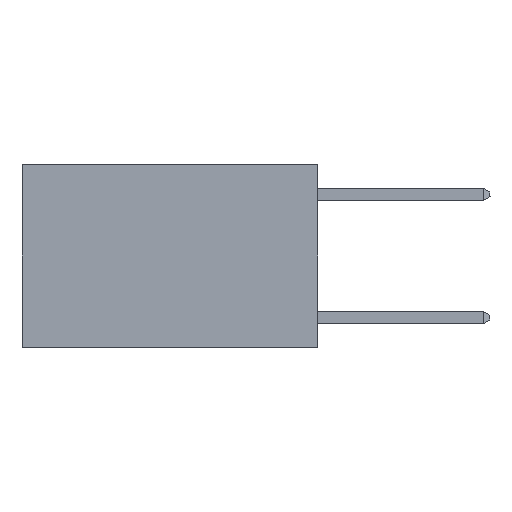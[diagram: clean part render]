
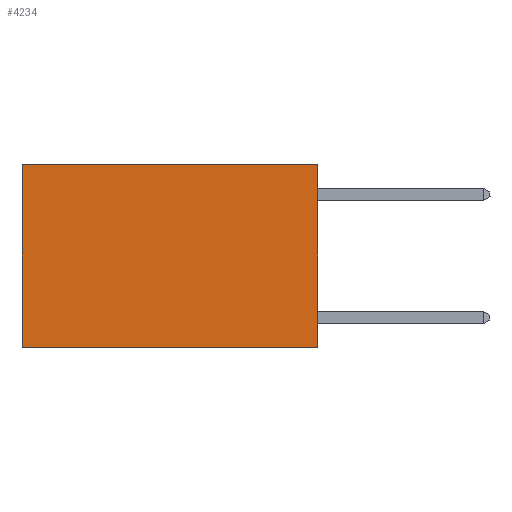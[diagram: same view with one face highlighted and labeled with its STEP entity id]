
A CAD part, left-side view. The second image highlights one B-rep face of the part: STEP entity #4234.
In plain terms, the highlighted planar face has unit normal (-1, 0, 0).
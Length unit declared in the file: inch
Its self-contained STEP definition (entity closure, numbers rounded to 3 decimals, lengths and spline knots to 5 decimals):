
#68 = VECTOR ( 'NONE', #19701, 39.37008 ) ;
#209 = CARTESIAN_POINT ( 'NONE',  ( 0.2625, 0., -0.37 ) ) ;
#572 = EDGE_CURVE ( 'NONE', #8072, #10551, #11175, .T. ) ;
#1167 = LINE ( 'NONE', #19522, #68 ) ;
#1258 = PLANE ( 'NONE',  #15353 ) ;
#1489 = DIRECTION ( 'NONE',  ( 0., 0., -1. ) ) ;
#2382 = CARTESIAN_POINT ( 'NONE',  ( 0.2625, 0.6, -0.37 ) ) ;
#2721 = ORIENTED_EDGE ( 'NONE', *, *, #7398, .T. ) ;
#2993 = CARTESIAN_POINT ( 'NONE',  ( 0.2625, 0., 0. ) ) ;
#3931 = VECTOR ( 'NONE', #5389, 39.37008 ) ;
#4234 = ADVANCED_FACE ( 'NONE', ( #5694 ), #1258, .F. ) ;
#5389 = DIRECTION ( 'NONE',  ( 0., 0., -1. ) ) ;
#5646 = ORIENTED_EDGE ( 'NONE', *, *, #14757, .F. ) ;
#5694 = FACE_OUTER_BOUND ( 'NONE', #10221, .T. ) ;
#5791 = DIRECTION ( 'NONE',  ( 1., 0., 0. ) ) ;
#6841 = CARTESIAN_POINT ( 'NONE',  ( 0.2625, 0.6, 0. ) ) ;
#6883 = LINE ( 'NONE', #19208, #3931 ) ;
#7398 = EDGE_CURVE ( 'NONE', #12377, #9652, #6883, .T. ) ;
#7489 = VECTOR ( 'NONE', #1489, 39.37008 ) ;
#7630 = CARTESIAN_POINT ( 'NONE',  ( 0.2625, 0., -0.37 ) ) ;
#8072 = VERTEX_POINT ( 'NONE', #14130 ) ;
#9652 = VERTEX_POINT ( 'NONE', #2382 ) ;
#10221 = EDGE_LOOP ( 'NONE', ( #2721, #5646, #16509, #12546 ) ) ;
#10551 = VERTEX_POINT ( 'NONE', #209 ) ;
#10674 = LINE ( 'NONE', #7630, #10773 ) ;
#10773 = VECTOR ( 'NONE', #12026, 39.37008 ) ;
#11175 = LINE ( 'NONE', #2993, #7489 ) ;
#11996 = DIRECTION ( 'NONE',  ( 0., 0., -1. ) ) ;
#12026 = DIRECTION ( 'NONE',  ( 0., 1., 0. ) ) ;
#12377 = VERTEX_POINT ( 'NONE', #6841 ) ;
#12546 = ORIENTED_EDGE ( 'NONE', *, *, #13730, .T. ) ;
#13730 = EDGE_CURVE ( 'NONE', #8072, #12377, #1167, .T. ) ;
#14130 = CARTESIAN_POINT ( 'NONE',  ( 0.2625, 0., 0. ) ) ;
#14757 = EDGE_CURVE ( 'NONE', #10551, #9652, #10674, .T. ) ;
#15353 = AXIS2_PLACEMENT_3D ( 'NONE', #16755, #5791, #11996 ) ;
#16509 = ORIENTED_EDGE ( 'NONE', *, *, #572, .F. ) ;
#16755 = CARTESIAN_POINT ( 'NONE',  ( 0.2625, 0., 0. ) ) ;
#19208 = CARTESIAN_POINT ( 'NONE',  ( 0.2625, 0.6, 0. ) ) ;
#19522 = CARTESIAN_POINT ( 'NONE',  ( 0.2625, 0., 0. ) ) ;
#19701 = DIRECTION ( 'NONE',  ( 0., 1., 0. ) ) ;
